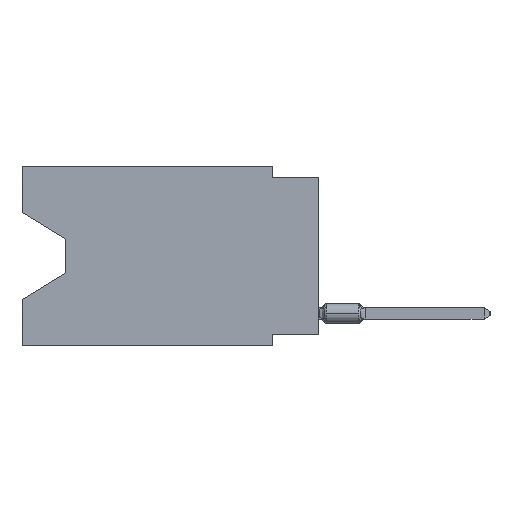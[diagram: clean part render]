
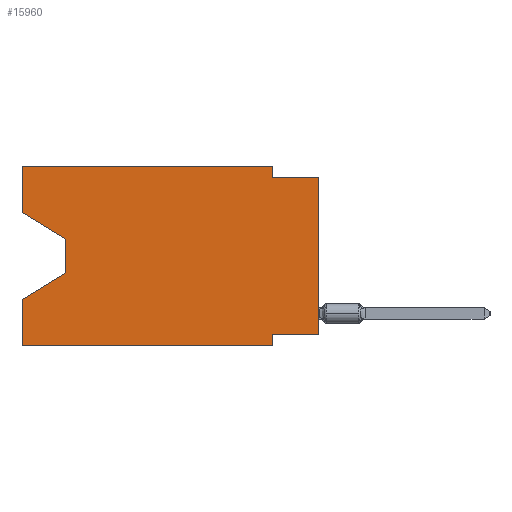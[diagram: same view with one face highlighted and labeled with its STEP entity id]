
A CAD part, left-side view. The second image highlights one B-rep face of the part: STEP entity #15960.
In plain terms, the highlighted planar face has unit normal (-1, 0, 0).
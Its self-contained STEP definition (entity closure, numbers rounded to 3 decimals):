
#330 = LINE ( 'NONE', #10337, #33246 ) ;
#786 = CARTESIAN_POINT ( 'NONE',  ( 0., 0., 0. ) ) ;
#1472 = LINE ( 'NONE', #11804, #26682 ) ;
#2948 = VECTOR ( 'NONE', #53806, 1000. ) ;
#3322 = LINE ( 'NONE', #14054, #19421 ) ;
#4216 = DIRECTION ( 'NONE',  ( 0., 0.855, -0.519 ) ) ;
#4801 = ORIENTED_EDGE ( 'NONE', *, *, #23628, .F. ) ;
#6010 = VECTOR ( 'NONE', #4216, 1000. ) ;
#6255 = DIRECTION ( 'NONE',  ( 0., 0., -1. ) ) ;
#6467 = EDGE_CURVE ( 'NONE', #16802, #14187, #24677, .T. ) ;
#8906 = LINE ( 'NONE', #38064, #42185 ) ;
#8969 = DIRECTION ( 'NONE',  ( 0., 0., -1. ) ) ;
#10337 = CARTESIAN_POINT ( 'NONE',  ( 0., 2.54, 0. ) ) ;
#11410 = DIRECTION ( 'NONE',  ( 0., -0.855, -0.519 ) ) ;
#11703 = CARTESIAN_POINT ( 'NONE',  ( 0., 0., -9.271 ) ) ;
#11804 = CARTESIAN_POINT ( 'NONE',  ( 0., 13.97, -4.013 ) ) ;
#12453 = EDGE_CURVE ( 'NONE', #15359, #15336, #32540, .T. ) ;
#12706 = CARTESIAN_POINT ( 'NONE',  ( 0., 16.383, -2.546 ) ) ;
#13951 = DIRECTION ( 'NONE',  ( 0., 0., 1. ) ) ;
#14054 = CARTESIAN_POINT ( 'NONE',  ( 0., 16.383, 0. ) ) ;
#14187 = VERTEX_POINT ( 'NONE', #21438 ) ;
#14589 = LINE ( 'NONE', #19770, #6010 ) ;
#15230 = LINE ( 'NONE', #20776, #21688 ) ;
#15336 = VERTEX_POINT ( 'NONE', #30479 ) ;
#15359 = VERTEX_POINT ( 'NONE', #35656 ) ;
#15865 = LINE ( 'NONE', #38041, #21109 ) ;
#15960 = ADVANCED_FACE ( 'NONE', ( #50869 ), #61957, .F. ) ;
#16607 = DIRECTION ( 'NONE',  ( 0., 0., -1. ) ) ;
#16802 = VERTEX_POINT ( 'NONE', #68449 ) ;
#16957 = CARTESIAN_POINT ( 'NONE',  ( 0., 2.54, 0. ) ) ;
#17410 = DIRECTION ( 'NONE',  ( 0., 0., 1. ) ) ;
#18056 = ORIENTED_EDGE ( 'NONE', *, *, #28908, .T. ) ;
#19133 = LINE ( 'NONE', #53095, #22290 ) ;
#19191 = CARTESIAN_POINT ( 'NONE',  ( 0., 13.97, -4.013 ) ) ;
#19421 = VECTOR ( 'NONE', #64661, 1000. ) ;
#19770 = CARTESIAN_POINT ( 'NONE',  ( 0., 13.97, -5.893 ) ) ;
#20370 = CARTESIAN_POINT ( 'NONE',  ( 0., 0., -0.635 ) ) ;
#20630 = EDGE_CURVE ( 'NONE', #16802, #52133, #3322, .T. ) ;
#20776 = CARTESIAN_POINT ( 'NONE',  ( 0., 2.54, -9.906 ) ) ;
#21109 = VECTOR ( 'NONE', #11410, 1000. ) ;
#21438 = CARTESIAN_POINT ( 'NONE',  ( 0., 2.54, -9.906 ) ) ;
#21454 = DIRECTION ( 'NONE',  ( 0., -1., 0. ) ) ;
#21688 = VECTOR ( 'NONE', #8969, 1000. ) ;
#22241 = AXIS2_PLACEMENT_3D ( 'NONE', #22818, #23933, #51617 ) ;
#22290 = VECTOR ( 'NONE', #13951, 1000. ) ;
#22568 = CARTESIAN_POINT ( 'NONE',  ( 0., 13.97, -5.893 ) ) ;
#22818 = CARTESIAN_POINT ( 'NONE',  ( 0., 16.383, 0. ) ) ;
#23600 = ORIENTED_EDGE ( 'NONE', *, *, #36426, .F. ) ;
#23628 = EDGE_CURVE ( 'NONE', #67683, #56675, #19133, .T. ) ;
#23933 = DIRECTION ( 'NONE',  ( 1., 0., 0. ) ) ;
#24677 = LINE ( 'NONE', #64539, #2948 ) ;
#25763 = CARTESIAN_POINT ( 'NONE',  ( 0., 0., -9.271 ) ) ;
#26412 = EDGE_CURVE ( 'NONE', #56496, #49733, #62294, .T. ) ;
#26682 = VECTOR ( 'NONE', #6255, 1000. ) ;
#28647 = CARTESIAN_POINT ( 'NONE',  ( 0., 16.383, -7.36 ) ) ;
#28908 = EDGE_CURVE ( 'NONE', #42650, #61629, #1472, .T. ) ;
#30479 = CARTESIAN_POINT ( 'NONE',  ( 0., 0., -0.635 ) ) ;
#31450 = DIRECTION ( 'NONE',  ( 0., -1., 0. ) ) ;
#32540 = LINE ( 'NONE', #20370, #33091 ) ;
#33066 = ORIENTED_EDGE ( 'NONE', *, *, #40307, .F. ) ;
#33091 = VECTOR ( 'NONE', #21454, 1000. ) ;
#33246 = VECTOR ( 'NONE', #16607, 1000. ) ;
#35656 = CARTESIAN_POINT ( 'NONE',  ( 0., 2.54, -0.635 ) ) ;
#36246 = ORIENTED_EDGE ( 'NONE', *, *, #54938, .T. ) ;
#36426 = EDGE_CURVE ( 'NONE', #56675, #68369, #8906, .T. ) ;
#37469 = EDGE_CURVE ( 'NONE', #49733, #14187, #15230, .T. ) ;
#38041 = CARTESIAN_POINT ( 'NONE',  ( 0., 16.383, -2.546 ) ) ;
#38064 = CARTESIAN_POINT ( 'NONE',  ( 0., 16.383, 0. ) ) ;
#39588 = LINE ( 'NONE', #786, #50773 ) ;
#40307 = EDGE_CURVE ( 'NONE', #68369, #15359, #330, .T. ) ;
#40531 = ORIENTED_EDGE ( 'NONE', *, *, #6467, .T. ) ;
#42185 = VECTOR ( 'NONE', #31450, 1000. ) ;
#42650 = VERTEX_POINT ( 'NONE', #19191 ) ;
#43084 = ORIENTED_EDGE ( 'NONE', *, *, #20630, .F. ) ;
#44594 = DIRECTION ( 'NONE',  ( 0., 1., 0. ) ) ;
#44906 = CARTESIAN_POINT ( 'NONE',  ( 0., 16.383, 0. ) ) ;
#45932 = CARTESIAN_POINT ( 'NONE',  ( 0., 2.54, -9.271 ) ) ;
#48384 = ORIENTED_EDGE ( 'NONE', *, *, #26412, .F. ) ;
#48413 = ORIENTED_EDGE ( 'NONE', *, *, #37469, .F. ) ;
#49300 = ORIENTED_EDGE ( 'NONE', *, *, #12453, .F. ) ;
#49733 = VERTEX_POINT ( 'NONE', #45932 ) ;
#50631 = ORIENTED_EDGE ( 'NONE', *, *, #51376, .T. ) ;
#50773 = VECTOR ( 'NONE', #17410, 1000. ) ;
#50869 = FACE_OUTER_BOUND ( 'NONE', #69257, .T. ) ;
#51376 = EDGE_CURVE ( 'NONE', #56496, #15336, #39588, .T. ) ;
#51617 = DIRECTION ( 'NONE',  ( 0., 0., -1. ) ) ;
#52133 = VERTEX_POINT ( 'NONE', #28647 ) ;
#53095 = CARTESIAN_POINT ( 'NONE',  ( 0., 16.383, 0. ) ) ;
#53806 = DIRECTION ( 'NONE',  ( 0., -1., 0. ) ) ;
#54938 = EDGE_CURVE ( 'NONE', #67683, #42650, #15865, .T. ) ;
#56496 = VERTEX_POINT ( 'NONE', #25763 ) ;
#56675 = VERTEX_POINT ( 'NONE', #44906 ) ;
#56936 = EDGE_CURVE ( 'NONE', #61629, #52133, #14589, .T. ) ;
#60718 = ORIENTED_EDGE ( 'NONE', *, *, #56936, .T. ) ;
#61629 = VERTEX_POINT ( 'NONE', #22568 ) ;
#61957 = PLANE ( 'NONE',  #22241 ) ;
#62294 = LINE ( 'NONE', #11703, #69158 ) ;
#64539 = CARTESIAN_POINT ( 'NONE',  ( 0., 16.383, -9.906 ) ) ;
#64661 = DIRECTION ( 'NONE',  ( 0., 0., 1. ) ) ;
#67683 = VERTEX_POINT ( 'NONE', #12706 ) ;
#68369 = VERTEX_POINT ( 'NONE', #16957 ) ;
#68449 = CARTESIAN_POINT ( 'NONE',  ( 0., 16.383, -9.906 ) ) ;
#69158 = VECTOR ( 'NONE', #44594, 1000. ) ;
#69257 = EDGE_LOOP ( 'NONE', ( #36246, #18056, #60718, #43084, #40531, #48413, #48384, #50631, #49300, #33066, #23600, #4801 ) ) ;
